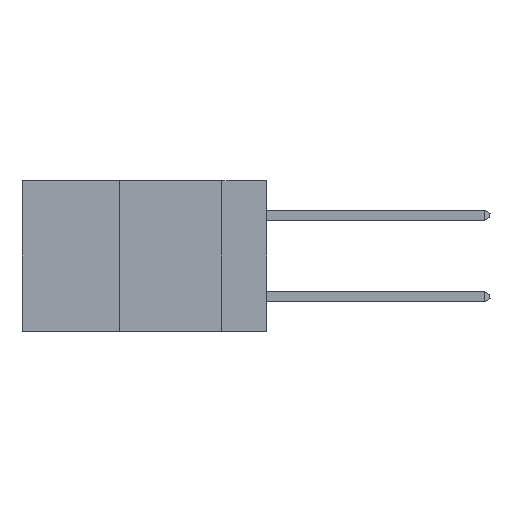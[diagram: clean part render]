
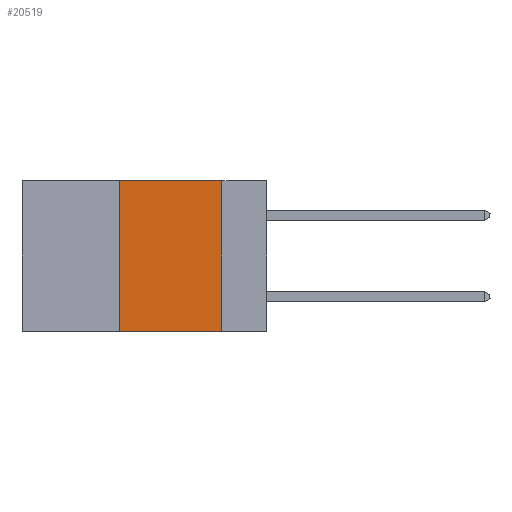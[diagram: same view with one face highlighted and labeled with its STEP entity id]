
A CAD part, left-side view. The second image highlights one B-rep face of the part: STEP entity #20519.
In plain terms, the highlighted planar face has unit normal (-1, 0, 0).
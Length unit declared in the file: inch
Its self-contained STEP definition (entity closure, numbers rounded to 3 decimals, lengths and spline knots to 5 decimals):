
#870 = ORIENTED_EDGE ( 'NONE', *, *, #10970, .T. ) ;
#1138 = LINE ( 'NONE', #22839, #17830 ) ;
#3139 = FACE_OUTER_BOUND ( 'NONE', #9067, .T. ) ;
#3818 = LINE ( 'NONE', #21521, #8491 ) ;
#3975 = VECTOR ( 'NONE', #12146, 39.37008 ) ;
#4833 = EDGE_CURVE ( 'NONE', #4908, #9683, #11145, .T. ) ;
#4908 = VERTEX_POINT ( 'NONE', #20742 ) ;
#5281 = DIRECTION ( 'NONE',  ( 1., 0., 0. ) ) ;
#5888 = VECTOR ( 'NONE', #22443, 39.37008 ) ;
#7361 = EDGE_CURVE ( 'NONE', #9683, #12487, #14460, .T. ) ;
#8308 = CARTESIAN_POINT ( 'NONE',  ( 0., 0.6, 0. ) ) ;
#8491 = VECTOR ( 'NONE', #17747, 39.37008 ) ;
#8975 = ORIENTED_EDGE ( 'NONE', *, *, #11572, .F. ) ;
#9067 = EDGE_LOOP ( 'NONE', ( #8975, #14164, #15992, #870 ) ) ;
#9683 = VERTEX_POINT ( 'NONE', #21409 ) ;
#10548 = CARTESIAN_POINT ( 'NONE',  ( 0., 0.11, 0. ) ) ;
#10970 = EDGE_CURVE ( 'NONE', #4908, #24682, #3818, .T. ) ;
#11144 = CARTESIAN_POINT ( 'NONE',  ( 0., 0.6, 0. ) ) ;
#11145 = LINE ( 'NONE', #20577, #5888 ) ;
#11304 = AXIS2_PLACEMENT_3D ( 'NONE', #11144, #5281, #19000 ) ;
#11572 = EDGE_CURVE ( 'NONE', #12487, #24682, #1138, .T. ) ;
#12146 = DIRECTION ( 'NONE',  ( 0., -1., 0. ) ) ;
#12487 = VERTEX_POINT ( 'NONE', #10548 ) ;
#14164 = ORIENTED_EDGE ( 'NONE', *, *, #7361, .F. ) ;
#14460 = LINE ( 'NONE', #8308, #3975 ) ;
#15992 = ORIENTED_EDGE ( 'NONE', *, *, #4833, .F. ) ;
#17747 = DIRECTION ( 'NONE',  ( 0., -1., 0. ) ) ;
#17830 = VECTOR ( 'NONE', #24769, 39.37008 ) ;
#18373 = CARTESIAN_POINT ( 'NONE',  ( 0., 0.11, -0.37 ) ) ;
#19000 = DIRECTION ( 'NONE',  ( 0., 0., -1. ) ) ;
#20519 = ADVANCED_FACE ( 'NONE', ( #3139 ), #20850, .F. ) ;
#20577 = CARTESIAN_POINT ( 'NONE',  ( 0., 0.36, 0. ) ) ;
#20742 = CARTESIAN_POINT ( 'NONE',  ( 0., 0.36, -0.37 ) ) ;
#20850 = PLANE ( 'NONE',  #11304 ) ;
#21409 = CARTESIAN_POINT ( 'NONE',  ( 0., 0.36, 0. ) ) ;
#21521 = CARTESIAN_POINT ( 'NONE',  ( 0., 0.6, -0.37 ) ) ;
#22443 = DIRECTION ( 'NONE',  ( 0., 0., 1. ) ) ;
#22839 = CARTESIAN_POINT ( 'NONE',  ( 0., 0.11, 0. ) ) ;
#24682 = VERTEX_POINT ( 'NONE', #18373 ) ;
#24769 = DIRECTION ( 'NONE',  ( 0., 0., -1. ) ) ;
